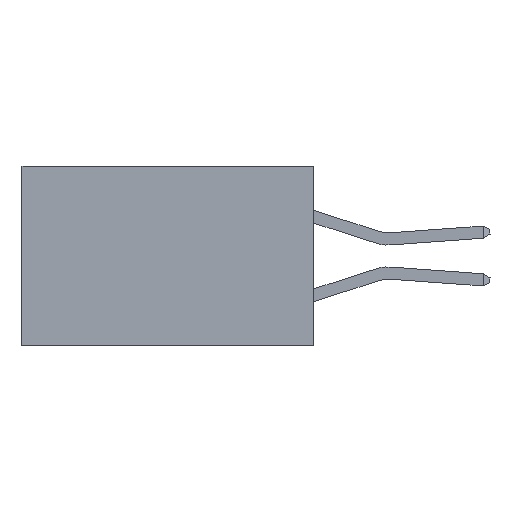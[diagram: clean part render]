
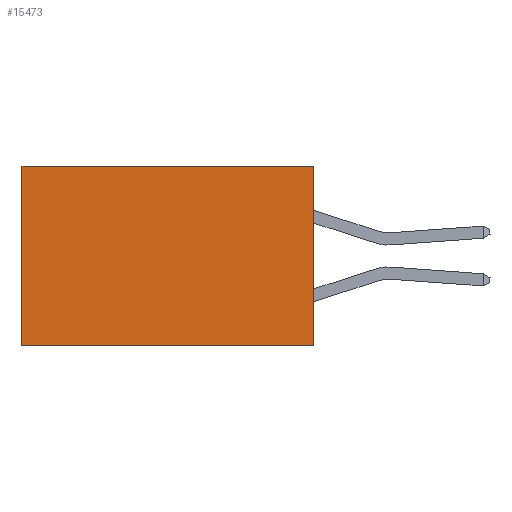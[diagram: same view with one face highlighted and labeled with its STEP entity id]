
A CAD part, left-side view. The second image highlights one B-rep face of the part: STEP entity #15473.
In plain terms, the highlighted planar face has unit normal (-1, 0, 0).
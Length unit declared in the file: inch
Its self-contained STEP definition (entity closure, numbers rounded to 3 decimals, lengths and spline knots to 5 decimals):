
#899 = VERTEX_POINT ( 'NONE', #9115 ) ;
#2164 = VECTOR ( 'NONE', #32168, 39.37008 ) ;
#2427 = VECTOR ( 'NONE', #20724, 39.37008 ) ;
#4128 = VERTEX_POINT ( 'NONE', #29625 ) ;
#4556 = ORIENTED_EDGE ( 'NONE', *, *, #17759, .F. ) ;
#5233 = VECTOR ( 'NONE', #6827, 39.37008 ) ;
#6827 = DIRECTION ( 'NONE',  ( 0., 1., 0. ) ) ;
#9115 = CARTESIAN_POINT ( 'NONE',  ( 0.2875, 0.6, -0.37 ) ) ;
#9310 = VECTOR ( 'NONE', #29320, 39.37008 ) ;
#9834 = CARTESIAN_POINT ( 'NONE',  ( 0.2875, 0., 0. ) ) ;
#9879 = ORIENTED_EDGE ( 'NONE', *, *, #32837, .T. ) ;
#10234 = VERTEX_POINT ( 'NONE', #25417 ) ;
#10309 = EDGE_LOOP ( 'NONE', ( #13429, #20773, #4556, #9879 ) ) ;
#10702 = LINE ( 'NONE', #12394, #2164 ) ;
#12019 = AXIS2_PLACEMENT_3D ( 'NONE', #9834, #15565, #35226 ) ;
#12394 = CARTESIAN_POINT ( 'NONE',  ( 0.2875, 0., 0. ) ) ;
#13429 = ORIENTED_EDGE ( 'NONE', *, *, #30218, .T. ) ;
#15473 = ADVANCED_FACE ( 'NONE', ( #19324 ), #32456, .F. ) ;
#15565 = DIRECTION ( 'NONE',  ( 1., 0., 0. ) ) ;
#15866 = LINE ( 'NONE', #26420, #2427 ) ;
#16913 = LINE ( 'NONE', #26470, #9310 ) ;
#17759 = EDGE_CURVE ( 'NONE', #31259, #10234, #10702, .T. ) ;
#19324 = FACE_OUTER_BOUND ( 'NONE', #10309, .T. ) ;
#20724 = DIRECTION ( 'NONE',  ( 0., 0., -1. ) ) ;
#20773 = ORIENTED_EDGE ( 'NONE', *, *, #20782, .F. ) ;
#20782 = EDGE_CURVE ( 'NONE', #10234, #899, #34425, .T. ) ;
#23833 = CARTESIAN_POINT ( 'NONE',  ( 0.2875, 0., -0.37 ) ) ;
#25417 = CARTESIAN_POINT ( 'NONE',  ( 0.2875, 0., -0.37 ) ) ;
#26420 = CARTESIAN_POINT ( 'NONE',  ( 0.2875, 0.6, 0. ) ) ;
#26470 = CARTESIAN_POINT ( 'NONE',  ( 0.2875, 0., 0. ) ) ;
#29320 = DIRECTION ( 'NONE',  ( 0., 1., 0. ) ) ;
#29625 = CARTESIAN_POINT ( 'NONE',  ( 0.2875, 0.6, 0. ) ) ;
#30218 = EDGE_CURVE ( 'NONE', #4128, #899, #15866, .T. ) ;
#31259 = VERTEX_POINT ( 'NONE', #33322 ) ;
#32168 = DIRECTION ( 'NONE',  ( 0., 0., -1. ) ) ;
#32456 = PLANE ( 'NONE',  #12019 ) ;
#32837 = EDGE_CURVE ( 'NONE', #31259, #4128, #16913, .T. ) ;
#33322 = CARTESIAN_POINT ( 'NONE',  ( 0.2875, 0., 0. ) ) ;
#34425 = LINE ( 'NONE', #23833, #5233 ) ;
#35226 = DIRECTION ( 'NONE',  ( 0., 0., -1. ) ) ;
